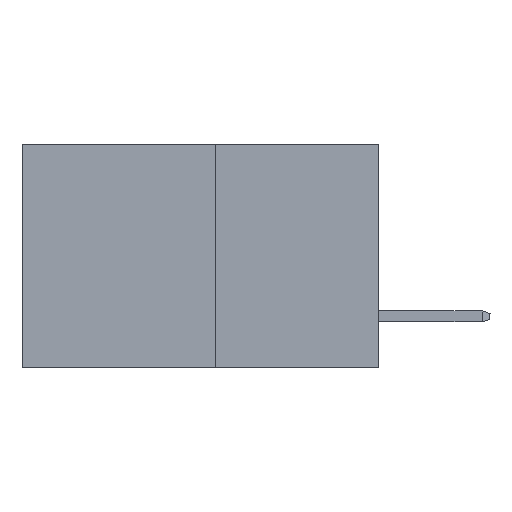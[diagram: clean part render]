
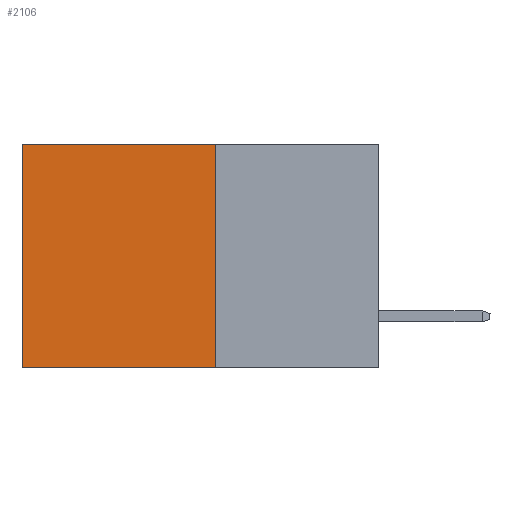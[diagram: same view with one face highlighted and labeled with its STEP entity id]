
A CAD part, left-side view. The second image highlights one B-rep face of the part: STEP entity #2106.
In plain terms, the highlighted planar face has unit normal (-1, 0, 0).
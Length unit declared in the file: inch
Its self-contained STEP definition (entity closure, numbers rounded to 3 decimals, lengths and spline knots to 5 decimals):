
#385 = EDGE_CURVE ( 'NONE', #4978, #2446, #4113, .T. ) ;
#536 = FACE_OUTER_BOUND ( 'NONE', #7758, .T. ) ;
#679 = VERTEX_POINT ( 'NONE', #820 ) ;
#802 = EDGE_CURVE ( 'NONE', #4978, #1744, #1670, .T. ) ;
#820 = CARTESIAN_POINT ( 'NONE',  ( 0.277, 0.59, -0.37 ) ) ;
#1398 = DIRECTION ( 'NONE',  ( 0., 0., -1. ) ) ;
#1614 = EDGE_CURVE ( 'NONE', #2446, #679, #6108, .T. ) ;
#1670 = LINE ( 'NONE', #7204, #5359 ) ;
#1730 = DIRECTION ( 'NONE',  ( 0., 0., -1. ) ) ;
#1744 = VERTEX_POINT ( 'NONE', #3777 ) ;
#1752 = DIRECTION ( 'NONE',  ( 1., 0., 0. ) ) ;
#1840 = ORIENTED_EDGE ( 'NONE', *, *, #3418, .F. ) ;
#2106 = ADVANCED_FACE ( 'NONE', ( #536 ), #9055, .F. ) ;
#2164 = VECTOR ( 'NONE', #2685, 39.37008 ) ;
#2223 = DIRECTION ( 'NONE',  ( 0., 1., 0. ) ) ;
#2446 = VERTEX_POINT ( 'NONE', #5926 ) ;
#2509 = VECTOR ( 'NONE', #1398, 39.37008 ) ;
#2685 = DIRECTION ( 'NONE',  ( 0., 1., 0. ) ) ;
#2792 = CARTESIAN_POINT ( 'NONE',  ( 0.277, 0.27, -0.37 ) ) ;
#2835 = VECTOR ( 'NONE', #2223, 39.37008 ) ;
#3019 = ORIENTED_EDGE ( 'NONE', *, *, #385, .T. ) ;
#3418 = EDGE_CURVE ( 'NONE', #1744, #679, #4535, .T. ) ;
#3777 = CARTESIAN_POINT ( 'NONE',  ( 0.277, 0.27, -0.37 ) ) ;
#4113 = LINE ( 'NONE', #4229, #2164 ) ;
#4229 = CARTESIAN_POINT ( 'NONE',  ( 0.277, 0.27, 0. ) ) ;
#4535 = LINE ( 'NONE', #2792, #2835 ) ;
#4978 = VERTEX_POINT ( 'NONE', #7083 ) ;
#5359 = VECTOR ( 'NONE', #5917, 39.37008 ) ;
#5631 = CARTESIAN_POINT ( 'NONE',  ( 0.277, 0.59, -0.37 ) ) ;
#5917 = DIRECTION ( 'NONE',  ( 0., 0., -1. ) ) ;
#5926 = CARTESIAN_POINT ( 'NONE',  ( 0.277, 0.59, 0. ) ) ;
#6108 = LINE ( 'NONE', #5631, #2509 ) ;
#7083 = CARTESIAN_POINT ( 'NONE',  ( 0.277, 0.27, 0. ) ) ;
#7204 = CARTESIAN_POINT ( 'NONE',  ( 0.277, 0.27, -0.37 ) ) ;
#7327 = CARTESIAN_POINT ( 'NONE',  ( 0.277, 0.27, -0.37 ) ) ;
#7632 = ORIENTED_EDGE ( 'NONE', *, *, #1614, .T. ) ;
#7758 = EDGE_LOOP ( 'NONE', ( #7632, #1840, #7929, #3019 ) ) ;
#7929 = ORIENTED_EDGE ( 'NONE', *, *, #802, .F. ) ;
#8398 = AXIS2_PLACEMENT_3D ( 'NONE', #7327, #1752, #1730 ) ;
#9055 = PLANE ( 'NONE',  #8398 ) ;
